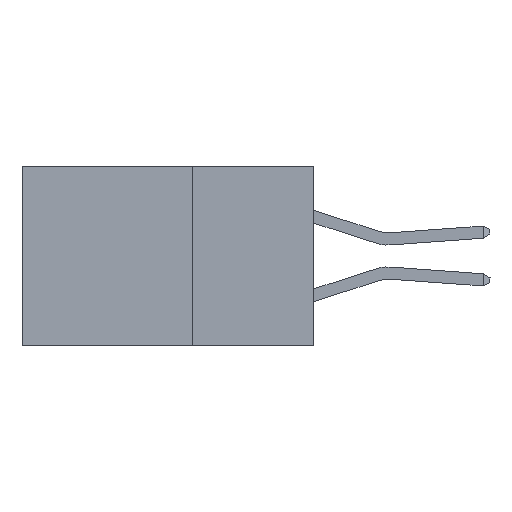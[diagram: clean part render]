
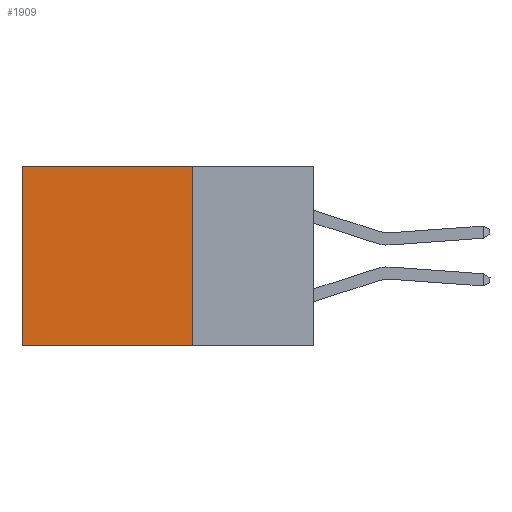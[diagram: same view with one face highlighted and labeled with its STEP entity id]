
A CAD part, left-side view. The second image highlights one B-rep face of the part: STEP entity #1909.
In plain terms, the highlighted planar face has unit normal (-1, 0, 0).
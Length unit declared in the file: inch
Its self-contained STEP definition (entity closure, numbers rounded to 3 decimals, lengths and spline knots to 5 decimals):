
#566 = EDGE_CURVE ( 'NONE', #12605, #11634, #2332, .T. ) ;
#1116 = CARTESIAN_POINT ( 'NONE',  ( 0.2875, 0.6, 0. ) ) ;
#1238 = VECTOR ( 'NONE', #22078, 39.37008 ) ;
#1582 = CARTESIAN_POINT ( 'NONE',  ( 0.2875, 0.6, 0. ) ) ;
#1909 = ADVANCED_FACE ( 'NONE', ( #3100 ), #15468, .F. ) ;
#2308 = LINE ( 'NONE', #16105, #22269 ) ;
#2332 = LINE ( 'NONE', #1116, #11113 ) ;
#2434 = LINE ( 'NONE', #6959, #3371 ) ;
#3100 = FACE_OUTER_BOUND ( 'NONE', #6042, .T. ) ;
#3371 = VECTOR ( 'NONE', #17308, 39.37008 ) ;
#3441 = LINE ( 'NONE', #9845, #1238 ) ;
#4801 = ORIENTED_EDGE ( 'NONE', *, *, #12155, .T. ) ;
#5919 = CARTESIAN_POINT ( 'NONE',  ( 0.2875, 0.6, -0.37 ) ) ;
#5976 = ORIENTED_EDGE ( 'NONE', *, *, #566, .T. ) ;
#6042 = EDGE_LOOP ( 'NONE', ( #5976, #13660, #9274, #4801 ) ) ;
#6959 = CARTESIAN_POINT ( 'NONE',  ( 0.2875, 0.25, -0.37 ) ) ;
#8536 = DIRECTION ( 'NONE',  ( 0., 0., -1. ) ) ;
#8773 = DIRECTION ( 'NONE',  ( 1., 0., 0. ) ) ;
#9274 = ORIENTED_EDGE ( 'NONE', *, *, #11291, .F. ) ;
#9845 = CARTESIAN_POINT ( 'NONE',  ( 0.2875, 0.25, 0. ) ) ;
#11113 = VECTOR ( 'NONE', #8536, 39.37008 ) ;
#11291 = EDGE_CURVE ( 'NONE', #15352, #16262, #3441, .T. ) ;
#11372 = CARTESIAN_POINT ( 'NONE',  ( 0.2875, 0.25, 0. ) ) ;
#11634 = VERTEX_POINT ( 'NONE', #5919 ) ;
#12155 = EDGE_CURVE ( 'NONE', #15352, #12605, #2308, .T. ) ;
#12605 = VERTEX_POINT ( 'NONE', #1582 ) ;
#13660 = ORIENTED_EDGE ( 'NONE', *, *, #22485, .F. ) ;
#13885 = DIRECTION ( 'NONE',  ( 0., 0., -1. ) ) ;
#15352 = VERTEX_POINT ( 'NONE', #11372 ) ;
#15468 = PLANE ( 'NONE',  #15701 ) ;
#15701 = AXIS2_PLACEMENT_3D ( 'NONE', #17239, #8773, #13885 ) ;
#15960 = CARTESIAN_POINT ( 'NONE',  ( 0.2875, 0.25, -0.37 ) ) ;
#16105 = CARTESIAN_POINT ( 'NONE',  ( 0.2875, 0.25, 0. ) ) ;
#16262 = VERTEX_POINT ( 'NONE', #15960 ) ;
#17239 = CARTESIAN_POINT ( 'NONE',  ( 0.2875, 0.25, 0. ) ) ;
#17308 = DIRECTION ( 'NONE',  ( 0., 1., 0. ) ) ;
#19660 = DIRECTION ( 'NONE',  ( 0., 1., 0. ) ) ;
#22078 = DIRECTION ( 'NONE',  ( 0., 0., -1. ) ) ;
#22269 = VECTOR ( 'NONE', #19660, 39.37008 ) ;
#22485 = EDGE_CURVE ( 'NONE', #16262, #11634, #2434, .T. ) ;
